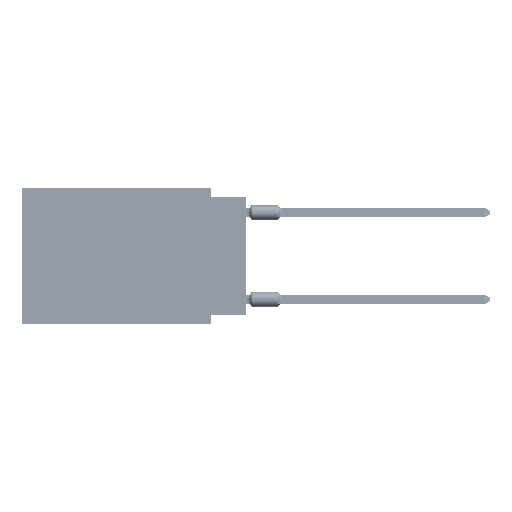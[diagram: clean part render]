
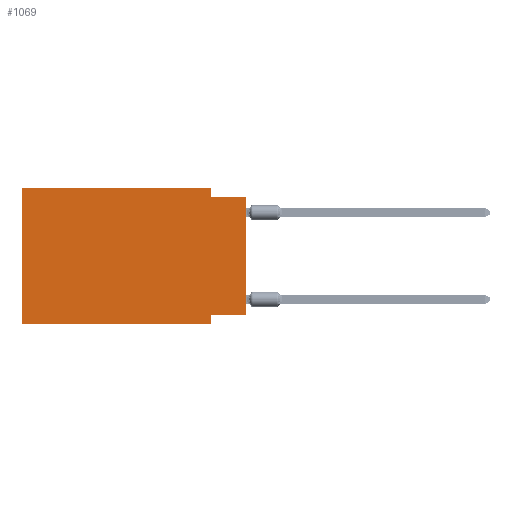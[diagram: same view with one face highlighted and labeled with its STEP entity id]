
A CAD part, left-side view. The second image highlights one B-rep face of the part: STEP entity #1069.
In plain terms, the highlighted planar face has unit normal (-1, 0, 0).
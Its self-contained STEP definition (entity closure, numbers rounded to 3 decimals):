
#220 = VERTEX_POINT ( 'NONE', #24564 ) ;
#1069 = ADVANCED_FACE ( 'NONE', ( #60722 ), #7282, .F. ) ;
#1566 = CARTESIAN_POINT ( 'NONE',  ( 0., 2.54, 0. ) ) ;
#1574 = ORIENTED_EDGE ( 'NONE', *, *, #43735, .T. ) ;
#2001 = EDGE_CURVE ( 'NONE', #20576, #220, #36377, .T. ) ;
#2263 = VECTOR ( 'NONE', #24727, 1000. ) ;
#2361 = ORIENTED_EDGE ( 'NONE', *, *, #15812, .F. ) ;
#2519 = EDGE_LOOP ( 'NONE', ( #1574, #15861, #64203, #18093, #2361, #5106, #38908, #13530 ) ) ;
#3336 = VERTEX_POINT ( 'NONE', #45197 ) ;
#5106 = ORIENTED_EDGE ( 'NONE', *, *, #2001, .T. ) ;
#6109 = EDGE_CURVE ( 'NONE', #33840, #41043, #52541, .T. ) ;
#6457 = CARTESIAN_POINT ( 'NONE',  ( 0., 2.54, -9.271 ) ) ;
#7282 = PLANE ( 'NONE',  #62758 ) ;
#7642 = CARTESIAN_POINT ( 'NONE',  ( 0., 16.383, 0. ) ) ;
#8141 = VECTOR ( 'NONE', #9106, 1000. ) ;
#8859 = DIRECTION ( 'NONE',  ( 0., 0., 1. ) ) ;
#9106 = DIRECTION ( 'NONE',  ( 0., -1., 0. ) ) ;
#11565 = CARTESIAN_POINT ( 'NONE',  ( 0., 0., 0. ) ) ;
#11687 = DIRECTION ( 'NONE',  ( 0., 0., -1. ) ) ;
#11836 = CARTESIAN_POINT ( 'NONE',  ( 0., 16.383, 0. ) ) ;
#13530 = ORIENTED_EDGE ( 'NONE', *, *, #6109, .F. ) ;
#15182 = CARTESIAN_POINT ( 'NONE',  ( 0., 0., -9.271 ) ) ;
#15812 = EDGE_CURVE ( 'NONE', #20576, #29500, #36126, .T. ) ;
#15861 = ORIENTED_EDGE ( 'NONE', *, *, #64151, .F. ) ;
#16112 = EDGE_CURVE ( 'NONE', #59220, #3336, #34053, .T. ) ;
#18093 = ORIENTED_EDGE ( 'NONE', *, *, #66125, .F. ) ;
#19342 = DIRECTION ( 'NONE',  ( 0., 1., 0. ) ) ;
#20576 = VERTEX_POINT ( 'NONE', #31528 ) ;
#22899 = CARTESIAN_POINT ( 'NONE',  ( 0., 2.54, -9.906 ) ) ;
#24564 = CARTESIAN_POINT ( 'NONE',  ( 0., 2.54, -9.906 ) ) ;
#24727 = DIRECTION ( 'NONE',  ( 0., 0., 1. ) ) ;
#27633 = LINE ( 'NONE', #11565, #2263 ) ;
#27660 = VECTOR ( 'NONE', #45017, 1000. ) ;
#28583 = EDGE_CURVE ( 'NONE', #41043, #220, #33063, .T. ) ;
#29287 = DIRECTION ( 'NONE',  ( 1., 0., 0. ) ) ;
#29500 = VERTEX_POINT ( 'NONE', #50005 ) ;
#30144 = CARTESIAN_POINT ( 'NONE',  ( 0., 0., -0.635 ) ) ;
#31528 = CARTESIAN_POINT ( 'NONE',  ( 0., 16.383, -9.906 ) ) ;
#33063 = LINE ( 'NONE', #22899, #41148 ) ;
#33840 = VERTEX_POINT ( 'NONE', #15182 ) ;
#34053 = LINE ( 'NONE', #1566, #36049 ) ;
#35410 = DIRECTION ( 'NONE',  ( 0., -1., 0. ) ) ;
#36049 = VECTOR ( 'NONE', #11687, 1000. ) ;
#36126 = LINE ( 'NONE', #51493, #37089 ) ;
#36377 = LINE ( 'NONE', #67778, #8141 ) ;
#37089 = VECTOR ( 'NONE', #8859, 1000. ) ;
#38908 = ORIENTED_EDGE ( 'NONE', *, *, #28583, .F. ) ;
#40308 = LINE ( 'NONE', #30144, #54141 ) ;
#41043 = VERTEX_POINT ( 'NONE', #6457 ) ;
#41148 = VECTOR ( 'NONE', #54716, 1000. ) ;
#43735 = EDGE_CURVE ( 'NONE', #33840, #45691, #27633, .T. ) ;
#44322 = LINE ( 'NONE', #7642, #27660 ) ;
#45017 = DIRECTION ( 'NONE',  ( 0., -1., 0. ) ) ;
#45197 = CARTESIAN_POINT ( 'NONE',  ( 0., 2.54, -0.635 ) ) ;
#45691 = VERTEX_POINT ( 'NONE', #47105 ) ;
#47105 = CARTESIAN_POINT ( 'NONE',  ( 0., 0., -0.635 ) ) ;
#50005 = CARTESIAN_POINT ( 'NONE',  ( 0., 16.383, 0. ) ) ;
#51493 = CARTESIAN_POINT ( 'NONE',  ( 0., 16.383, 0. ) ) ;
#51838 = CARTESIAN_POINT ( 'NONE',  ( 0., 0., -9.271 ) ) ;
#52541 = LINE ( 'NONE', #51838, #63223 ) ;
#54141 = VECTOR ( 'NONE', #35410, 1000. ) ;
#54716 = DIRECTION ( 'NONE',  ( 0., 0., -1. ) ) ;
#56634 = CARTESIAN_POINT ( 'NONE',  ( 0., 2.54, 0. ) ) ;
#59220 = VERTEX_POINT ( 'NONE', #56634 ) ;
#60722 = FACE_OUTER_BOUND ( 'NONE', #2519, .T. ) ;
#61073 = DIRECTION ( 'NONE',  ( 0., 0., -1. ) ) ;
#62758 = AXIS2_PLACEMENT_3D ( 'NONE', #11836, #29287, #61073 ) ;
#63223 = VECTOR ( 'NONE', #19342, 1000. ) ;
#64151 = EDGE_CURVE ( 'NONE', #3336, #45691, #40308, .T. ) ;
#64203 = ORIENTED_EDGE ( 'NONE', *, *, #16112, .F. ) ;
#66125 = EDGE_CURVE ( 'NONE', #29500, #59220, #44322, .T. ) ;
#67778 = CARTESIAN_POINT ( 'NONE',  ( 0., 16.383, -9.906 ) ) ;
